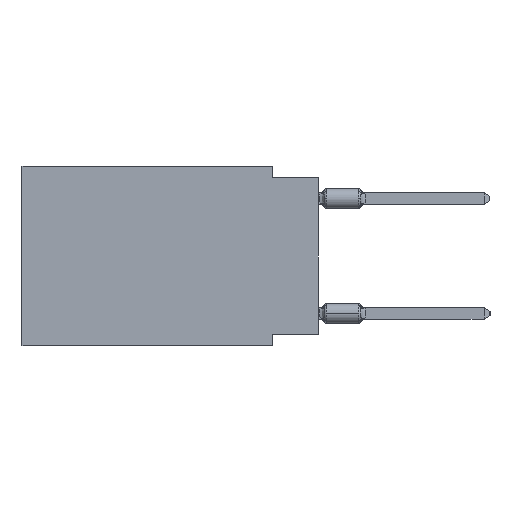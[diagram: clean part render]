
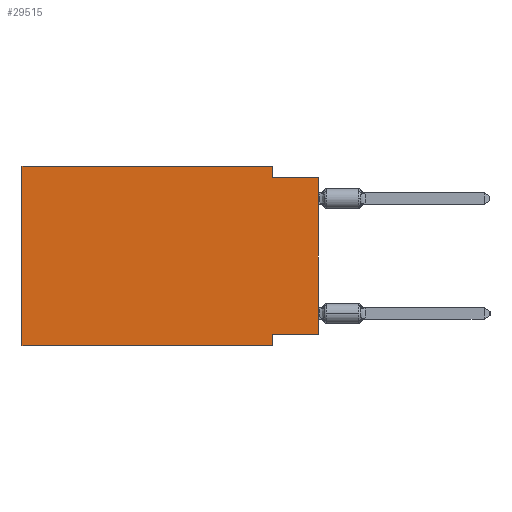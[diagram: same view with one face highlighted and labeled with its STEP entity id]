
A CAD part, left-side view. The second image highlights one B-rep face of the part: STEP entity #29515.
In plain terms, the highlighted planar face has unit normal (-1, 0, 0).
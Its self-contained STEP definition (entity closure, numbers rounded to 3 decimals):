
#439 = DIRECTION ( 'NONE',  ( 0., 0., -1. ) ) ;
#452 = EDGE_CURVE ( 'NONE', #45479, #27312, #12586, .T. ) ;
#546 = EDGE_CURVE ( 'NONE', #1276, #33614, #36798, .T. ) ;
#1276 = VERTEX_POINT ( 'NONE', #39340 ) ;
#1940 = EDGE_CURVE ( 'NONE', #33614, #7725, #51424, .T. ) ;
#1983 = CARTESIAN_POINT ( 'NONE',  ( 0., 2.54, -9.271 ) ) ;
#3308 = VECTOR ( 'NONE', #44929, 1000. ) ;
#4641 = CARTESIAN_POINT ( 'NONE',  ( 0., 16.383, 0. ) ) ;
#6539 = EDGE_CURVE ( 'NONE', #9479, #27312, #27567, .T. ) ;
#7080 = DIRECTION ( 'NONE',  ( 0., 0., -1. ) ) ;
#7629 = DIRECTION ( 'NONE',  ( 1., 0., 0. ) ) ;
#7725 = VERTEX_POINT ( 'NONE', #14919 ) ;
#8540 = CARTESIAN_POINT ( 'NONE',  ( 0., 16.383, -9.906 ) ) ;
#9479 = VERTEX_POINT ( 'NONE', #20984 ) ;
#9810 = DIRECTION ( 'NONE',  ( 0., -1., 0. ) ) ;
#10254 = ORIENTED_EDGE ( 'NONE', *, *, #1940, .F. ) ;
#10612 = VECTOR ( 'NONE', #439, 1000. ) ;
#11156 = FACE_OUTER_BOUND ( 'NONE', #30075, .T. ) ;
#11740 = DIRECTION ( 'NONE',  ( 0., 0., -1. ) ) ;
#12432 = VECTOR ( 'NONE', #28378, 1000. ) ;
#12586 = LINE ( 'NONE', #15588, #21072 ) ;
#12898 = EDGE_CURVE ( 'NONE', #19061, #29981, #16709, .T. ) ;
#14537 = CARTESIAN_POINT ( 'NONE',  ( 0., 16.383, 0. ) ) ;
#14919 = CARTESIAN_POINT ( 'NONE',  ( 0., 2.54, 0. ) ) ;
#15097 = VECTOR ( 'NONE', #43536, 1000. ) ;
#15588 = CARTESIAN_POINT ( 'NONE',  ( 0., 0., 0. ) ) ;
#15853 = DIRECTION ( 'NONE',  ( 0., 0., 1. ) ) ;
#16531 = VECTOR ( 'NONE', #50798, 1000. ) ;
#16709 = LINE ( 'NONE', #33243, #10612 ) ;
#19008 = ORIENTED_EDGE ( 'NONE', *, *, #6539, .F. ) ;
#19061 = VERTEX_POINT ( 'NONE', #1983 ) ;
#19595 = AXIS2_PLACEMENT_3D ( 'NONE', #44771, #7629, #7080 ) ;
#20984 = CARTESIAN_POINT ( 'NONE',  ( 0., 2.54, -0.635 ) ) ;
#21072 = VECTOR ( 'NONE', #15853, 1000. ) ;
#22057 = CARTESIAN_POINT ( 'NONE',  ( 0., 0., -9.271 ) ) ;
#22584 = LINE ( 'NONE', #22057, #16531 ) ;
#23142 = LINE ( 'NONE', #44281, #33212 ) ;
#23470 = ORIENTED_EDGE ( 'NONE', *, *, #45946, .F. ) ;
#23507 = CARTESIAN_POINT ( 'NONE',  ( 0., 0., -0.635 ) ) ;
#26273 = CARTESIAN_POINT ( 'NONE',  ( 0., 0., -9.271 ) ) ;
#26592 = EDGE_CURVE ( 'NONE', #45479, #19061, #22584, .T. ) ;
#27312 = VERTEX_POINT ( 'NONE', #53388 ) ;
#27567 = LINE ( 'NONE', #23507, #3308 ) ;
#27674 = PLANE ( 'NONE',  #19595 ) ;
#28378 = DIRECTION ( 'NONE',  ( 0., 0., 1. ) ) ;
#28585 = LINE ( 'NONE', #8540, #47056 ) ;
#29515 = ADVANCED_FACE ( 'NONE', ( #11156 ), #27674, .F. ) ;
#29981 = VERTEX_POINT ( 'NONE', #30232 ) ;
#30075 = EDGE_LOOP ( 'NONE', ( #40415, #19008, #23470, #10254, #43568, #47035, #49341, #49293 ) ) ;
#30232 = CARTESIAN_POINT ( 'NONE',  ( 0., 2.54, -9.906 ) ) ;
#33212 = VECTOR ( 'NONE', #11740, 1000. ) ;
#33243 = CARTESIAN_POINT ( 'NONE',  ( 0., 2.54, -9.906 ) ) ;
#33614 = VERTEX_POINT ( 'NONE', #4641 ) ;
#35987 = CARTESIAN_POINT ( 'NONE',  ( 0., 16.383, 0. ) ) ;
#36798 = LINE ( 'NONE', #35987, #12432 ) ;
#38428 = EDGE_CURVE ( 'NONE', #1276, #29981, #28585, .T. ) ;
#39340 = CARTESIAN_POINT ( 'NONE',  ( 0., 16.383, -9.906 ) ) ;
#40415 = ORIENTED_EDGE ( 'NONE', *, *, #452, .T. ) ;
#43536 = DIRECTION ( 'NONE',  ( 0., -1., 0. ) ) ;
#43568 = ORIENTED_EDGE ( 'NONE', *, *, #546, .F. ) ;
#44281 = CARTESIAN_POINT ( 'NONE',  ( 0., 2.54, 0. ) ) ;
#44771 = CARTESIAN_POINT ( 'NONE',  ( 0., 16.383, 0. ) ) ;
#44929 = DIRECTION ( 'NONE',  ( 0., -1., 0. ) ) ;
#45479 = VERTEX_POINT ( 'NONE', #26273 ) ;
#45946 = EDGE_CURVE ( 'NONE', #7725, #9479, #23142, .T. ) ;
#47035 = ORIENTED_EDGE ( 'NONE', *, *, #38428, .T. ) ;
#47056 = VECTOR ( 'NONE', #9810, 1000. ) ;
#49293 = ORIENTED_EDGE ( 'NONE', *, *, #26592, .F. ) ;
#49341 = ORIENTED_EDGE ( 'NONE', *, *, #12898, .F. ) ;
#50798 = DIRECTION ( 'NONE',  ( 0., 1., 0. ) ) ;
#51424 = LINE ( 'NONE', #14537, #15097 ) ;
#53388 = CARTESIAN_POINT ( 'NONE',  ( 0., 0., -0.635 ) ) ;
